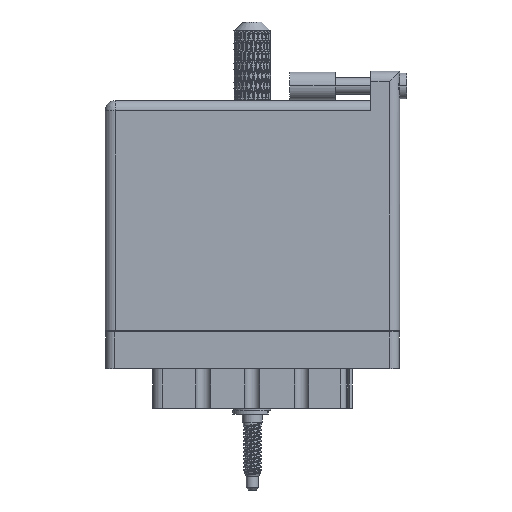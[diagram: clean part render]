
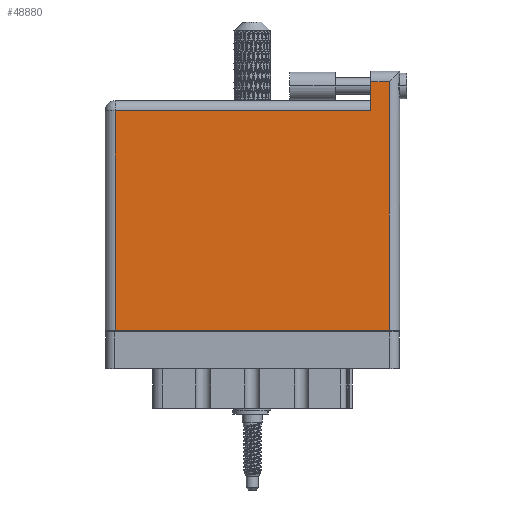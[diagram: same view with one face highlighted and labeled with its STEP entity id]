
A CAD part, front view. The second image highlights one B-rep face of the part: STEP entity #48880.
In plain terms, the highlighted face is planar.
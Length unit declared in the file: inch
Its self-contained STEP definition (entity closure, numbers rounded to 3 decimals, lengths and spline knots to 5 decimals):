
#1134 = AXIS2_PLACEMENT_3D ( 'NONE', #51265, #84232, #43201 ) ;
#1208 = CARTESIAN_POINT ( 'NONE',  ( 1.811, 1.496, 0. ) ) ;
#4209 = FACE_OUTER_BOUND ( 'NONE', #57836, .T. ) ;
#8981 = LINE ( 'NONE', #65221, #56377 ) ;
#10121 = DIRECTION ( 'NONE',  ( 0., -1., 0. ) ) ;
#11212 = VERTEX_POINT ( 'NONE', #67110 ) ;
#12365 = ORIENTED_EDGE ( 'NONE', *, *, #65664, .T. ) ;
#18755 = CARTESIAN_POINT ( 'NONE',  ( 0.07, 0., 0. ) ) ;
#27510 = PLANE ( 'NONE',  #1134 ) ;
#27801 = DIRECTION ( 'NONE',  ( -1., 0., 0. ) ) ;
#28404 = EDGE_CURVE ( 'NONE', #99620, #63021, #52245, .T. ) ;
#29388 = VECTOR ( 'NONE', #10121, 39.37008 ) ;
#29699 = DIRECTION ( 'NONE',  ( 0., 1., 0. ) ) ;
#31134 = EDGE_CURVE ( 'NONE', #40564, #11212, #62353, .T. ) ;
#32893 = VECTOR ( 'NONE', #94641, 39.37008 ) ;
#34302 = EDGE_CURVE ( 'NONE', #11212, #41288, #50007, .T. ) ;
#35664 = LINE ( 'NONE', #68586, #102177 ) ;
#38096 = CARTESIAN_POINT ( 'NONE',  ( 0., 1.696, 0. ) ) ;
#40564 = VERTEX_POINT ( 'NONE', #78427 ) ;
#41288 = VERTEX_POINT ( 'NONE', #1208 ) ;
#41379 = ORIENTED_EDGE ( 'NONE', *, *, #80794, .T. ) ;
#43201 = DIRECTION ( 'NONE',  ( -1., 0., 0. ) ) ;
#48880 = ADVANCED_FACE ( 'NONE', ( #4209 ), #27510, .F. ) ;
#50007 = LINE ( 'NONE', #67799, #70530 ) ;
#50090 = ORIENTED_EDGE ( 'NONE', *, *, #28404, .T. ) ;
#51265 = CARTESIAN_POINT ( 'NONE',  ( 0., 1.566, 0. ) ) ;
#51584 = DIRECTION ( 'NONE',  ( 0., -1., 0. ) ) ;
#52245 = LINE ( 'NONE', #18755, #29388 ) ;
#55632 = CARTESIAN_POINT ( 'NONE',  ( 0.07, 1.496, 0. ) ) ;
#56377 = VECTOR ( 'NONE', #91631, 39.37008 ) ;
#57836 = EDGE_LOOP ( 'NONE', ( #41379, #12365, #84106, #104045, #84180, #50090 ) ) ;
#59113 = EDGE_CURVE ( 'NONE', #41288, #99620, #62761, .T. ) ;
#60911 = VERTEX_POINT ( 'NONE', #92032 ) ;
#62353 = LINE ( 'NONE', #38096, #67485 ) ;
#62761 = LINE ( 'NONE', #86001, #32893 ) ;
#63021 = VERTEX_POINT ( 'NONE', #79640 ) ;
#65221 = CARTESIAN_POINT ( 'NONE',  ( 0., 0., 0. ) ) ;
#65664 = EDGE_CURVE ( 'NONE', #60911, #40564, #35664, .T. ) ;
#67110 = CARTESIAN_POINT ( 'NONE',  ( 1.811, 1.696, 0. ) ) ;
#67485 = VECTOR ( 'NONE', #27801, 39.37008 ) ;
#67799 = CARTESIAN_POINT ( 'NONE',  ( 1.811, 1.766, 0. ) ) ;
#68586 = CARTESIAN_POINT ( 'NONE',  ( 1.938, 1.766, 0. ) ) ;
#70530 = VECTOR ( 'NONE', #51584, 39.37008 ) ;
#78427 = CARTESIAN_POINT ( 'NONE',  ( 1.938, 1.696, 0. ) ) ;
#79640 = CARTESIAN_POINT ( 'NONE',  ( 0.07, 0., 0. ) ) ;
#80794 = EDGE_CURVE ( 'NONE', #63021, #60911, #8981, .T. ) ;
#84106 = ORIENTED_EDGE ( 'NONE', *, *, #31134, .T. ) ;
#84180 = ORIENTED_EDGE ( 'NONE', *, *, #59113, .T. ) ;
#84232 = DIRECTION ( 'NONE',  ( 0., 0., -1. ) ) ;
#86001 = CARTESIAN_POINT ( 'NONE',  ( 0., 1.496, 0. ) ) ;
#91631 = DIRECTION ( 'NONE',  ( 1., 0., 0. ) ) ;
#92032 = CARTESIAN_POINT ( 'NONE',  ( 1.938, 0., 0. ) ) ;
#94641 = DIRECTION ( 'NONE',  ( -1., 0., 0. ) ) ;
#99620 = VERTEX_POINT ( 'NONE', #55632 ) ;
#102177 = VECTOR ( 'NONE', #29699, 39.37008 ) ;
#104045 = ORIENTED_EDGE ( 'NONE', *, *, #34302, .T. ) ;
